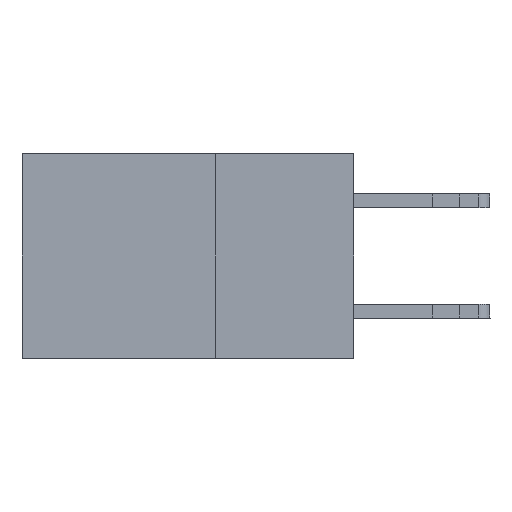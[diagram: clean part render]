
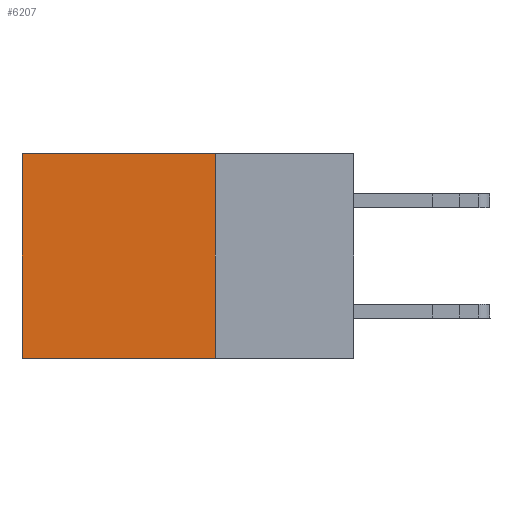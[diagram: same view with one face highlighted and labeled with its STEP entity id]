
A CAD part, left-side view. The second image highlights one B-rep face of the part: STEP entity #6207.
In plain terms, the highlighted planar face has unit normal (-1, 0, 0).
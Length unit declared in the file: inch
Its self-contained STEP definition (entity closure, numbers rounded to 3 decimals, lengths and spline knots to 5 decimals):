
#451 = LINE ( 'NONE', #10868, #22812 ) ;
#1358 = ORIENTED_EDGE ( 'NONE', *, *, #5968, .T. ) ;
#1725 = VERTEX_POINT ( 'NONE', #15137 ) ;
#2893 = CARTESIAN_POINT ( 'NONE',  ( 0.2875, 0.25, 0. ) ) ;
#3232 = CARTESIAN_POINT ( 'NONE',  ( 0.2875, 0.6, -0.37 ) ) ;
#3863 = DIRECTION ( 'NONE',  ( 0., 1., 0. ) ) ;
#4294 = VERTEX_POINT ( 'NONE', #16953 ) ;
#4632 = CARTESIAN_POINT ( 'NONE',  ( 0.2875, 0.25, 0. ) ) ;
#5800 = CARTESIAN_POINT ( 'NONE',  ( 0.2875, 0.25, 0. ) ) ;
#5968 = EDGE_CURVE ( 'NONE', #22200, #12683, #12497, .T. ) ;
#6207 = ADVANCED_FACE ( 'NONE', ( #6461 ), #10977, .F. ) ;
#6360 = ORIENTED_EDGE ( 'NONE', *, *, #16302, .F. ) ;
#6416 = DIRECTION ( 'NONE',  ( 0., 1., 0. ) ) ;
#6461 = FACE_OUTER_BOUND ( 'NONE', #20014, .T. ) ;
#6526 = DIRECTION ( 'NONE',  ( 0., 0., -1. ) ) ;
#7183 = ORIENTED_EDGE ( 'NONE', *, *, #7397, .F. ) ;
#7397 = EDGE_CURVE ( 'NONE', #4294, #12683, #451, .T. ) ;
#7531 = DIRECTION ( 'NONE',  ( 0., 0., -1. ) ) ;
#8431 = VECTOR ( 'NONE', #6526, 39.37008 ) ;
#8474 = VECTOR ( 'NONE', #6416, 39.37008 ) ;
#10868 = CARTESIAN_POINT ( 'NONE',  ( 0.2875, 0.25, -0.37 ) ) ;
#10977 = PLANE ( 'NONE',  #18531 ) ;
#11936 = VECTOR ( 'NONE', #13764, 39.37008 ) ;
#12421 = CARTESIAN_POINT ( 'NONE',  ( 0.2875, 0.6, 0. ) ) ;
#12497 = LINE ( 'NONE', #20729, #11936 ) ;
#12683 = VERTEX_POINT ( 'NONE', #3232 ) ;
#13591 = EDGE_CURVE ( 'NONE', #1725, #22200, #22922, .T. ) ;
#13764 = DIRECTION ( 'NONE',  ( 0., 0., -1. ) ) ;
#15137 = CARTESIAN_POINT ( 'NONE',  ( 0.2875, 0.25, 0. ) ) ;
#16302 = EDGE_CURVE ( 'NONE', #1725, #4294, #22324, .T. ) ;
#16953 = CARTESIAN_POINT ( 'NONE',  ( 0.2875, 0.25, -0.37 ) ) ;
#18057 = DIRECTION ( 'NONE',  ( 1., 0., 0. ) ) ;
#18531 = AXIS2_PLACEMENT_3D ( 'NONE', #5800, #18057, #7531 ) ;
#20014 = EDGE_LOOP ( 'NONE', ( #1358, #7183, #6360, #21610 ) ) ;
#20729 = CARTESIAN_POINT ( 'NONE',  ( 0.2875, 0.6, 0. ) ) ;
#21610 = ORIENTED_EDGE ( 'NONE', *, *, #13591, .T. ) ;
#22200 = VERTEX_POINT ( 'NONE', #12421 ) ;
#22324 = LINE ( 'NONE', #2893, #8431 ) ;
#22812 = VECTOR ( 'NONE', #3863, 39.37008 ) ;
#22922 = LINE ( 'NONE', #4632, #8474 ) ;
